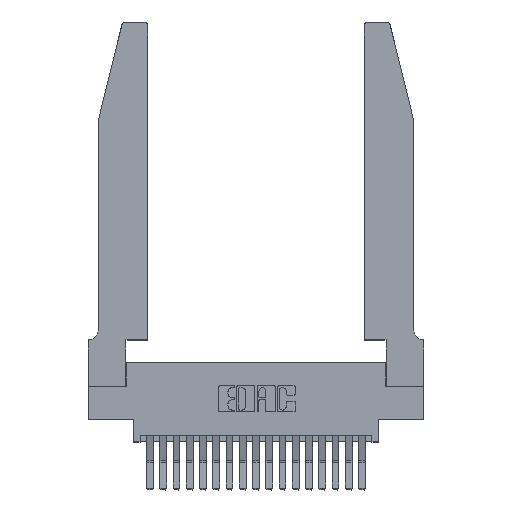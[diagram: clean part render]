
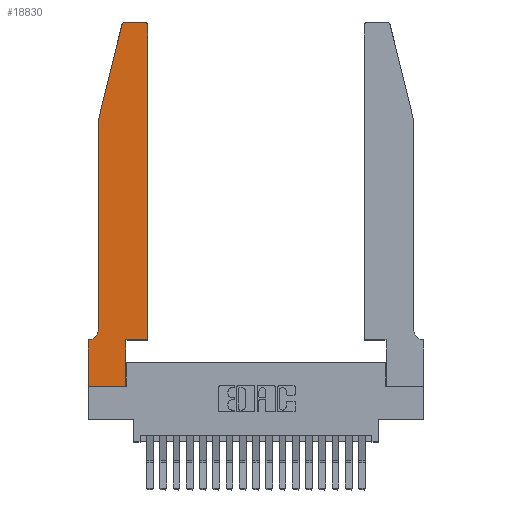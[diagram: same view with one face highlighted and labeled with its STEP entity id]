
A CAD part, top view. The second image highlights one B-rep face of the part: STEP entity #18830.
In plain terms, the highlighted planar face has unit normal (0, 0, 1).
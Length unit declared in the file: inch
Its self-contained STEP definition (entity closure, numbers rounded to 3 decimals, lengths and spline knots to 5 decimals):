
#593 = PLANE ( 'NONE',  #14896 ) ;
#841 = DIRECTION ( 'NONE',  ( 0., 0., 1. ) ) ;
#1710 = CARTESIAN_POINT ( 'NONE',  ( 0.2865, 0., 0.37 ) ) ;
#1806 = DIRECTION ( 'NONE',  ( 0., 0., -1. ) ) ;
#1808 = CARTESIAN_POINT ( 'NONE',  ( 0.4505, 2.72, 0.37 ) ) ;
#2281 = CARTESIAN_POINT ( 'NONE',  ( 0., 0.35, 0.37 ) ) ;
#2301 = LINE ( 'NONE', #11100, #17500 ) ;
#2362 = DIRECTION ( 'NONE',  ( 1., 0., 0. ) ) ;
#2393 = VECTOR ( 'NONE', #17458, 39.37008 ) ;
#2503 = EDGE_CURVE ( 'NONE', #14897, #16153, #4544, .T. ) ;
#2535 = EDGE_CURVE ( 'NONE', #7756, #4434, #8738, .T. ) ;
#3270 = ORIENTED_EDGE ( 'NONE', *, *, #15639, .T. ) ;
#3634 = DIRECTION ( 'NONE',  ( 1., 0., 0. ) ) ;
#3773 = CARTESIAN_POINT ( 'NONE',  ( 0.4205, 2.72, 0.37 ) ) ;
#3795 = CARTESIAN_POINT ( 'NONE',  ( 0.25487, 2.72718, 0.37 ) ) ;
#3972 = DIRECTION ( 'NONE',  ( 0., 0., 1. ) ) ;
#4434 = VERTEX_POINT ( 'NONE', #3795 ) ;
#4544 = LINE ( 'NONE', #16003, #13432 ) ;
#5175 = AXIS2_PLACEMENT_3D ( 'NONE', #13481, #1806, #13268 ) ;
#5459 = ORIENTED_EDGE ( 'NONE', *, *, #13868, .T. ) ;
#5707 = DIRECTION ( 'NONE',  ( 1., 0., 0. ) ) ;
#5847 = EDGE_CURVE ( 'NONE', #19692, #9006, #14656, .T. ) ;
#6410 = CARTESIAN_POINT ( 'NONE',  ( 0.4205, 2.75, 0.37 ) ) ;
#6539 = DIRECTION ( 'NONE',  ( -0.239, -0.971, 0. ) ) ;
#6835 = EDGE_CURVE ( 'NONE', #9006, #7756, #12232, .T. ) ;
#6846 = ORIENTED_EDGE ( 'NONE', *, *, #18862, .T. ) ;
#7267 = DIRECTION ( 'NONE',  ( 0., 1., 0. ) ) ;
#7756 = VERTEX_POINT ( 'NONE', #11603 ) ;
#7871 = ORIENTED_EDGE ( 'NONE', *, *, #6835, .T. ) ;
#8448 = CIRCLE ( 'NONE', #5175, 0.07 ) ;
#8738 = CIRCLE ( 'NONE', #17934, 0.03 ) ;
#8835 = LINE ( 'NONE', #15887, #17725 ) ;
#8989 = VERTEX_POINT ( 'NONE', #18389 ) ;
#9006 = VERTEX_POINT ( 'NONE', #6410 ) ;
#9121 = DIRECTION ( 'NONE',  ( 1., 0., 0. ) ) ;
#9888 = DIRECTION ( 'NONE',  ( 0., 1., 0. ) ) ;
#10104 = CARTESIAN_POINT ( 'NONE',  ( 0.2605, 2.75, 0.37 ) ) ;
#10379 = VECTOR ( 'NONE', #7267, 39.37008 ) ;
#10586 = EDGE_CURVE ( 'NONE', #18175, #17241, #2301, .T. ) ;
#10695 = VERTEX_POINT ( 'NONE', #11069 ) ;
#10921 = CARTESIAN_POINT ( 'NONE',  ( 0., 0., 0.37 ) ) ;
#11069 = CARTESIAN_POINT ( 'NONE',  ( 0.0055, 0.35, 0.37 ) ) ;
#11100 = CARTESIAN_POINT ( 'NONE',  ( 0.0755, 2., 0.37 ) ) ;
#11295 = LINE ( 'NONE', #10921, #2393 ) ;
#11462 = CARTESIAN_POINT ( 'NONE',  ( 0.4505, 0.35, 0.37 ) ) ;
#11603 = CARTESIAN_POINT ( 'NONE',  ( 0.284, 2.75, 0.37 ) ) ;
#11681 = ORIENTED_EDGE ( 'NONE', *, *, #19969, .T. ) ;
#11689 = VECTOR ( 'NONE', #6539, 39.37008 ) ;
#11964 = EDGE_LOOP ( 'NONE', ( #7871, #16901, #14867, #18587, #3270, #13893, #21508, #14423, #5459, #6846, #11681, #13547 ) ) ;
#12055 = EDGE_CURVE ( 'NONE', #4434, #18175, #16146, .T. ) ;
#12232 = LINE ( 'NONE', #10104, #18797 ) ;
#12511 = CARTESIAN_POINT ( 'NONE',  ( 0., 0., 0.37 ) ) ;
#12615 = DIRECTION ( 'NONE',  ( 1., 0., 0. ) ) ;
#13268 = DIRECTION ( 'NONE',  ( -1., 0., 0. ) ) ;
#13432 = VECTOR ( 'NONE', #12615, 39.37008 ) ;
#13481 = CARTESIAN_POINT ( 'NONE',  ( 0.0055, 0.42, 0.37 ) ) ;
#13547 = ORIENTED_EDGE ( 'NONE', *, *, #5847, .T. ) ;
#13833 = LINE ( 'NONE', #16526, #16466 ) ;
#13868 = EDGE_CURVE ( 'NONE', #16153, #8989, #16858, .T. ) ;
#13893 = ORIENTED_EDGE ( 'NONE', *, *, #17497, .T. ) ;
#14423 = ORIENTED_EDGE ( 'NONE', *, *, #2503, .T. ) ;
#14561 = FACE_OUTER_BOUND ( 'NONE', #11964, .T. ) ;
#14656 = CIRCLE ( 'NONE', #19644, 0.03 ) ;
#14867 = ORIENTED_EDGE ( 'NONE', *, *, #12055, .T. ) ;
#14896 = AXIS2_PLACEMENT_3D ( 'NONE', #2281, #3972, #5707 ) ;
#14897 = VERTEX_POINT ( 'NONE', #12511 ) ;
#15498 = DIRECTION ( 'NONE',  ( 0., 0., 1. ) ) ;
#15561 = VERTEX_POINT ( 'NONE', #11462 ) ;
#15639 = EDGE_CURVE ( 'NONE', #17241, #10695, #8448, .T. ) ;
#15887 = CARTESIAN_POINT ( 'NONE',  ( 0.4505, 0.35, 0.37 ) ) ;
#15918 = CARTESIAN_POINT ( 'NONE',  ( 0., 0.35, 0.37 ) ) ;
#15932 = EDGE_CURVE ( 'NONE', #21479, #14897, #11295, .T. ) ;
#16003 = CARTESIAN_POINT ( 'NONE',  ( 0., 0., 0.37 ) ) ;
#16146 = LINE ( 'NONE', #21626, #11689 ) ;
#16153 = VERTEX_POINT ( 'NONE', #1710 ) ;
#16466 = VECTOR ( 'NONE', #19992, 39.37008 ) ;
#16526 = CARTESIAN_POINT ( 'NONE',  ( 0.0755, 0.35, 0.37 ) ) ;
#16858 = LINE ( 'NONE', #21308, #18156 ) ;
#16901 = ORIENTED_EDGE ( 'NONE', *, *, #2535, .T. ) ;
#17241 = VERTEX_POINT ( 'NONE', #21278 ) ;
#17458 = DIRECTION ( 'NONE',  ( 0., -1., 0. ) ) ;
#17497 = EDGE_CURVE ( 'NONE', #10695, #21479, #13833, .T. ) ;
#17500 = VECTOR ( 'NONE', #21199, 39.37008 ) ;
#17725 = VECTOR ( 'NONE', #2362, 39.37008 ) ;
#17934 = AXIS2_PLACEMENT_3D ( 'NONE', #19159, #841, #9121 ) ;
#18156 = VECTOR ( 'NONE', #9888, 39.37008 ) ;
#18175 = VERTEX_POINT ( 'NONE', #18829 ) ;
#18389 = CARTESIAN_POINT ( 'NONE',  ( 0.2865, 0.35, 0.37 ) ) ;
#18587 = ORIENTED_EDGE ( 'NONE', *, *, #10586, .T. ) ;
#18797 = VECTOR ( 'NONE', #20158, 39.37008 ) ;
#18829 = CARTESIAN_POINT ( 'NONE',  ( 0.0755, 2., 0.37 ) ) ;
#18830 = ADVANCED_FACE ( 'NONE', ( #14561 ), #593, .T. ) ;
#18862 = EDGE_CURVE ( 'NONE', #8989, #15561, #8835, .T. ) ;
#18924 = CARTESIAN_POINT ( 'NONE',  ( 0.4505, 0.35, 0.37 ) ) ;
#19159 = CARTESIAN_POINT ( 'NONE',  ( 0.284, 2.72, 0.37 ) ) ;
#19282 = LINE ( 'NONE', #18924, #10379 ) ;
#19644 = AXIS2_PLACEMENT_3D ( 'NONE', #3773, #15498, #3634 ) ;
#19692 = VERTEX_POINT ( 'NONE', #1808 ) ;
#19969 = EDGE_CURVE ( 'NONE', #15561, #19692, #19282, .T. ) ;
#19992 = DIRECTION ( 'NONE',  ( -1., 0., 0. ) ) ;
#20158 = DIRECTION ( 'NONE',  ( -1., 0., 0. ) ) ;
#21199 = DIRECTION ( 'NONE',  ( 0., -1., 0. ) ) ;
#21278 = CARTESIAN_POINT ( 'NONE',  ( 0.0755, 0.42, 0.37 ) ) ;
#21308 = CARTESIAN_POINT ( 'NONE',  ( 0.2865, 0.35, 0.37 ) ) ;
#21479 = VERTEX_POINT ( 'NONE', #15918 ) ;
#21508 = ORIENTED_EDGE ( 'NONE', *, *, #15932, .T. ) ;
#21626 = CARTESIAN_POINT ( 'NONE',  ( 0.0755, 2., 0.37 ) ) ;
